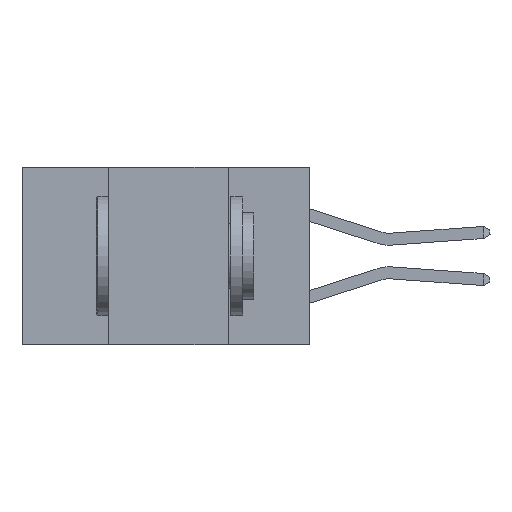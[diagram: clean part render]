
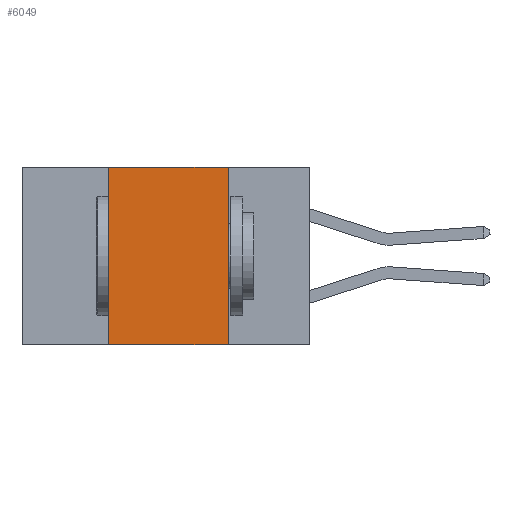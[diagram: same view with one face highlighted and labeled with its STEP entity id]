
A CAD part, left-side view. The second image highlights one B-rep face of the part: STEP entity #6049.
In plain terms, the highlighted planar face has unit normal (-1, 0, 0).
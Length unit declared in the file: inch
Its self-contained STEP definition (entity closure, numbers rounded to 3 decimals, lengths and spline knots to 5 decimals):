
#293 = LINE ( 'NONE', #13331, #13622 ) ;
#322 = VECTOR ( 'NONE', #6730, 39.37008 ) ;
#443 = DIRECTION ( 'NONE',  ( 0., -1., 0. ) ) ;
#852 = ORIENTED_EDGE ( 'NONE', *, *, #11935, .T. ) ;
#1232 = CARTESIAN_POINT ( 'NONE',  ( 0., 0.17, 0. ) ) ;
#2115 = AXIS2_PLACEMENT_3D ( 'NONE', #5904, #3577, #3582 ) ;
#2784 = CARTESIAN_POINT ( 'NONE',  ( 0., 0.17, -0.37 ) ) ;
#3262 = VECTOR ( 'NONE', #443, 39.37008 ) ;
#3577 = DIRECTION ( 'NONE',  ( 1., 0., 0. ) ) ;
#3582 = DIRECTION ( 'NONE',  ( 0., 0., -1. ) ) ;
#4966 = ORIENTED_EDGE ( 'NONE', *, *, #14118, .F. ) ;
#4989 = CARTESIAN_POINT ( 'NONE',  ( 0., 0.6, 0. ) ) ;
#5904 = CARTESIAN_POINT ( 'NONE',  ( 0., 0.6, 0. ) ) ;
#6049 = ADVANCED_FACE ( 'NONE', ( #10150 ), #15099, .F. ) ;
#6730 = DIRECTION ( 'NONE',  ( 0., -1., 0. ) ) ;
#7429 = VERTEX_POINT ( 'NONE', #16857 ) ;
#7449 = VERTEX_POINT ( 'NONE', #1232 ) ;
#9588 = LINE ( 'NONE', #4989, #322 ) ;
#10150 = FACE_OUTER_BOUND ( 'NONE', #20717, .T. ) ;
#10343 = EDGE_CURVE ( 'NONE', #13928, #7429, #293, .T. ) ;
#11935 = EDGE_CURVE ( 'NONE', #13928, #22064, #21702, .T. ) ;
#13331 = CARTESIAN_POINT ( 'NONE',  ( 0., 0.42, 0. ) ) ;
#13622 = VECTOR ( 'NONE', #18578, 39.37008 ) ;
#13928 = VERTEX_POINT ( 'NONE', #21415 ) ;
#14118 = EDGE_CURVE ( 'NONE', #7429, #7449, #9588, .T. ) ;
#14165 = ORIENTED_EDGE ( 'NONE', *, *, #10343, .F. ) ;
#15024 = EDGE_CURVE ( 'NONE', #7449, #22064, #19683, .T. ) ;
#15099 = PLANE ( 'NONE',  #2115 ) ;
#15807 = CARTESIAN_POINT ( 'NONE',  ( 0., 0.17, 0. ) ) ;
#16857 = CARTESIAN_POINT ( 'NONE',  ( 0., 0.42, 0. ) ) ;
#17593 = DIRECTION ( 'NONE',  ( 0., 0., -1. ) ) ;
#18578 = DIRECTION ( 'NONE',  ( 0., 0., 1. ) ) ;
#19150 = VECTOR ( 'NONE', #17593, 39.37008 ) ;
#19582 = CARTESIAN_POINT ( 'NONE',  ( 0., 0.6, -0.37 ) ) ;
#19683 = LINE ( 'NONE', #15807, #19150 ) ;
#20717 = EDGE_LOOP ( 'NONE', ( #21206, #4966, #14165, #852 ) ) ;
#21206 = ORIENTED_EDGE ( 'NONE', *, *, #15024, .F. ) ;
#21415 = CARTESIAN_POINT ( 'NONE',  ( 0., 0.42, -0.37 ) ) ;
#21702 = LINE ( 'NONE', #19582, #3262 ) ;
#22064 = VERTEX_POINT ( 'NONE', #2784 ) ;
